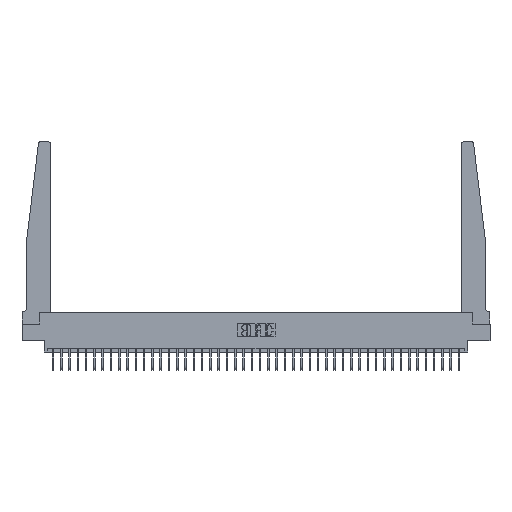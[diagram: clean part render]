
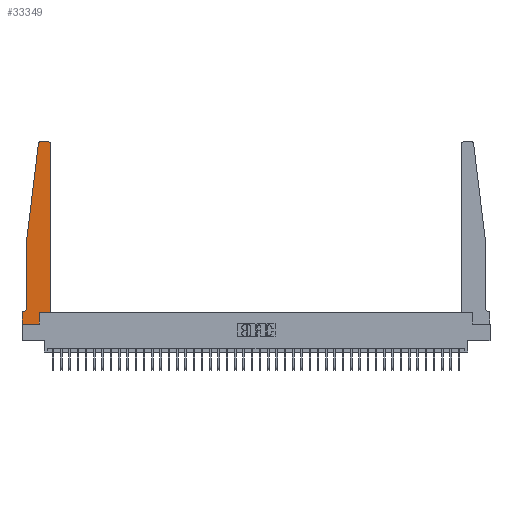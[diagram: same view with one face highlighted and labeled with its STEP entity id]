
A CAD part, top view. The second image highlights one B-rep face of the part: STEP entity #33349.
In plain terms, the highlighted planar face has unit normal (0, 0, 1).
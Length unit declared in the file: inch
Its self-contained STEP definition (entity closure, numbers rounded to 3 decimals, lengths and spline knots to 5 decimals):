
#314 = LINE ( 'NONE', #27457, #28189 ) ;
#341 = DIRECTION ( 'NONE',  ( 0., 0., -1. ) ) ;
#765 = PLANE ( 'NONE',  #16554 ) ;
#796 = ORIENTED_EDGE ( 'NONE', *, *, #4478, .T. ) ;
#2040 = DIRECTION ( 'NONE',  ( -0.122, -0.992, 0. ) ) ;
#3024 = VERTEX_POINT ( 'NONE', #25489 ) ;
#3298 = ORIENTED_EDGE ( 'NONE', *, *, #13949, .T. ) ;
#3409 = AXIS2_PLACEMENT_3D ( 'NONE', #16491, #341, #19208 ) ;
#3451 = DIRECTION ( 'NONE',  ( 1., 0., 0. ) ) ;
#3685 = AXIS2_PLACEMENT_3D ( 'NONE', #28733, #12507, #31440 ) ;
#3798 = EDGE_CURVE ( 'NONE', #9788, #10721, #27845, .T. ) ;
#4116 = LINE ( 'NONE', #14233, #31975 ) ;
#4206 = VERTEX_POINT ( 'NONE', #14163 ) ;
#4478 = EDGE_CURVE ( 'NONE', #10221, #10691, #20172, .T. ) ;
#6195 = VECTOR ( 'NONE', #10273, 39.37008 ) ;
#6232 = DIRECTION ( 'NONE',  ( 0., 1., 0. ) ) ;
#9025 = DIRECTION ( 'NONE',  ( 0., 1., 0. ) ) ;
#9515 = VERTEX_POINT ( 'NONE', #11345 ) ;
#9528 = CARTESIAN_POINT ( 'NONE',  ( 0.065, 1.25, 0.37 ) ) ;
#9788 = VERTEX_POINT ( 'NONE', #20774 ) ;
#10221 = VERTEX_POINT ( 'NONE', #9528 ) ;
#10273 = DIRECTION ( 'NONE',  ( 0., -1., 0. ) ) ;
#10691 = VERTEX_POINT ( 'NONE', #16968 ) ;
#10721 = VERTEX_POINT ( 'NONE', #25180 ) ;
#10956 = VECTOR ( 'NONE', #16975, 39.37008 ) ;
#11345 = CARTESIAN_POINT ( 'NONE',  ( 0.425, 0.18, 0.37 ) ) ;
#11362 = AXIS2_PLACEMENT_3D ( 'NONE', #15326, #34173, #18047 ) ;
#11451 = LINE ( 'NONE', #28429, #19500 ) ;
#11506 = LINE ( 'NONE', #18201, #25870 ) ;
#11672 = EDGE_CURVE ( 'NONE', #19120, #28772, #13370, .T. ) ;
#12507 = DIRECTION ( 'NONE',  ( 0., 0., 1. ) ) ;
#13367 = CARTESIAN_POINT ( 'NONE',  ( 0., 0., 0.37 ) ) ;
#13370 = LINE ( 'NONE', #18427, #6195 ) ;
#13849 = EDGE_CURVE ( 'NONE', #3024, #19120, #314, .T. ) ;
#13949 = EDGE_CURVE ( 'NONE', #9515, #9788, #4116, .T. ) ;
#14163 = CARTESIAN_POINT ( 'NONE',  ( 0.27653, 2.75, 0.37 ) ) ;
#14233 = CARTESIAN_POINT ( 'NONE',  ( 0.425, 0.18, 0.37 ) ) ;
#14810 = FACE_OUTER_BOUND ( 'NONE', #33451, .T. ) ;
#15326 = CARTESIAN_POINT ( 'NONE',  ( 0.27653, 2.72, 0.37 ) ) ;
#15558 = EDGE_CURVE ( 'NONE', #4206, #19240, #27640, .T. ) ;
#15842 = ORIENTED_EDGE ( 'NONE', *, *, #21583, .T. ) ;
#15887 = CARTESIAN_POINT ( 'NONE',  ( 0., 0.1875, 0.37 ) ) ;
#16359 = CARTESIAN_POINT ( 'NONE',  ( 0.24675, 2.72367, 0.37 ) ) ;
#16491 = CARTESIAN_POINT ( 'NONE',  ( 0.015, 0.2375, 0.37 ) ) ;
#16554 = AXIS2_PLACEMENT_3D ( 'NONE', #22190, #19624, #3451 ) ;
#16966 = EDGE_CURVE ( 'NONE', #19240, #10221, #11506, .T. ) ;
#16968 = CARTESIAN_POINT ( 'NONE',  ( 0.065, 0.2375, 0.37 ) ) ;
#16975 = DIRECTION ( 'NONE',  ( 1., 0., 0. ) ) ;
#17162 = ORIENTED_EDGE ( 'NONE', *, *, #16966, .T. ) ;
#17171 = EDGE_CURVE ( 'NONE', #19013, #30350, #27995, .T. ) ;
#17315 = LINE ( 'NONE', #33128, #10956 ) ;
#18047 = DIRECTION ( 'NONE',  ( 1., 0., 0. ) ) ;
#18201 = CARTESIAN_POINT ( 'NONE',  ( 0.065, 1.25, 0.37 ) ) ;
#18427 = CARTESIAN_POINT ( 'NONE',  ( 0., 0., 0.37 ) ) ;
#18463 = VECTOR ( 'NONE', #34462, 39.37008 ) ;
#18572 = ORIENTED_EDGE ( 'NONE', *, *, #28288, .T. ) ;
#18888 = EDGE_CURVE ( 'NONE', #30350, #9515, #11451, .T. ) ;
#19013 = VERTEX_POINT ( 'NONE', #28904 ) ;
#19120 = VERTEX_POINT ( 'NONE', #15887 ) ;
#19208 = DIRECTION ( 'NONE',  ( -1., 0., 0. ) ) ;
#19240 = VERTEX_POINT ( 'NONE', #16359 ) ;
#19500 = VECTOR ( 'NONE', #33810, 39.37008 ) ;
#19624 = DIRECTION ( 'NONE',  ( 0., 0., 1. ) ) ;
#19945 = VECTOR ( 'NONE', #6232, 39.37008 ) ;
#20172 = LINE ( 'NONE', #28817, #33679 ) ;
#20348 = ORIENTED_EDGE ( 'NONE', *, *, #15558, .T. ) ;
#20774 = CARTESIAN_POINT ( 'NONE',  ( 0.425, 2.72, 0.37 ) ) ;
#21583 = EDGE_CURVE ( 'NONE', #10721, #4206, #25607, .T. ) ;
#22190 = CARTESIAN_POINT ( 'NONE',  ( 0., 0.1875, 0.37 ) ) ;
#23894 = CARTESIAN_POINT ( 'NONE',  ( 0.2605, 0.18, 0.37 ) ) ;
#24968 = CIRCLE ( 'NONE', #3409, 0.05 ) ;
#24992 = CARTESIAN_POINT ( 'NONE',  ( 0.2605, 0.18, 0.37 ) ) ;
#25116 = ORIENTED_EDGE ( 'NONE', *, *, #3798, .T. ) ;
#25180 = CARTESIAN_POINT ( 'NONE',  ( 0.395, 2.75, 0.37 ) ) ;
#25489 = CARTESIAN_POINT ( 'NONE',  ( 0.015, 0.1875, 0.37 ) ) ;
#25607 = LINE ( 'NONE', #29207, #18463 ) ;
#25870 = VECTOR ( 'NONE', #2040, 39.37008 ) ;
#26844 = ORIENTED_EDGE ( 'NONE', *, *, #11672, .T. ) ;
#27457 = CARTESIAN_POINT ( 'NONE',  ( 0.065, 0.1875, 0.37 ) ) ;
#27640 = CIRCLE ( 'NONE', #11362, 0.03 ) ;
#27845 = CIRCLE ( 'NONE', #3685, 0.03 ) ;
#27995 = LINE ( 'NONE', #24992, #19945 ) ;
#28189 = VECTOR ( 'NONE', #32888, 39.37008 ) ;
#28288 = EDGE_CURVE ( 'NONE', #28772, #19013, #17315, .T. ) ;
#28429 = CARTESIAN_POINT ( 'NONE',  ( 0.425, 0.18, 0.37 ) ) ;
#28733 = CARTESIAN_POINT ( 'NONE',  ( 0.395, 2.72, 0.37 ) ) ;
#28772 = VERTEX_POINT ( 'NONE', #13367 ) ;
#28817 = CARTESIAN_POINT ( 'NONE',  ( 0.065, 1.25, 0.37 ) ) ;
#28904 = CARTESIAN_POINT ( 'NONE',  ( 0.2605, 0., 0.37 ) ) ;
#29207 = CARTESIAN_POINT ( 'NONE',  ( 0.25, 2.75, 0.37 ) ) ;
#29743 = ORIENTED_EDGE ( 'NONE', *, *, #32559, .T. ) ;
#30350 = VERTEX_POINT ( 'NONE', #23894 ) ;
#31161 = ORIENTED_EDGE ( 'NONE', *, *, #18888, .T. ) ;
#31440 = DIRECTION ( 'NONE',  ( 1., 0., 0. ) ) ;
#31523 = DIRECTION ( 'NONE',  ( 0., -1., 0. ) ) ;
#31975 = VECTOR ( 'NONE', #9025, 39.37008 ) ;
#32213 = ORIENTED_EDGE ( 'NONE', *, *, #13849, .T. ) ;
#32559 = EDGE_CURVE ( 'NONE', #10691, #3024, #24968, .T. ) ;
#32888 = DIRECTION ( 'NONE',  ( -1., 0., 0. ) ) ;
#33128 = CARTESIAN_POINT ( 'NONE',  ( 0., 0., 0.37 ) ) ;
#33349 = ADVANCED_FACE ( 'NONE', ( #14810 ), #765, .T. ) ;
#33451 = EDGE_LOOP ( 'NONE', ( #15842, #20348, #17162, #796, #29743, #32213, #26844, #18572, #34656, #31161, #3298, #25116 ) ) ;
#33679 = VECTOR ( 'NONE', #31523, 39.37008 ) ;
#33810 = DIRECTION ( 'NONE',  ( 1., 0., 0. ) ) ;
#34173 = DIRECTION ( 'NONE',  ( 0., 0., 1. ) ) ;
#34462 = DIRECTION ( 'NONE',  ( -1., 0., 0. ) ) ;
#34656 = ORIENTED_EDGE ( 'NONE', *, *, #17171, .T. ) ;
